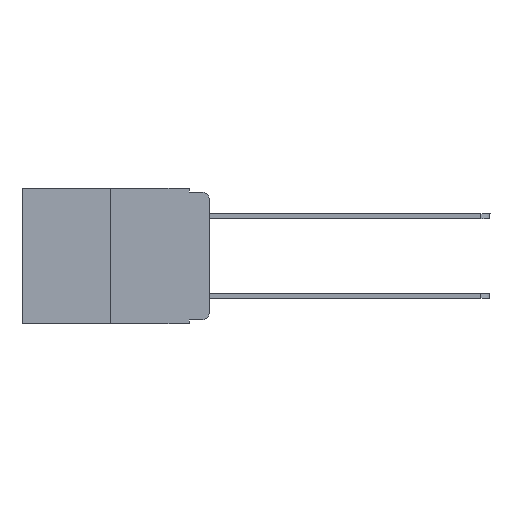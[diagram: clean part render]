
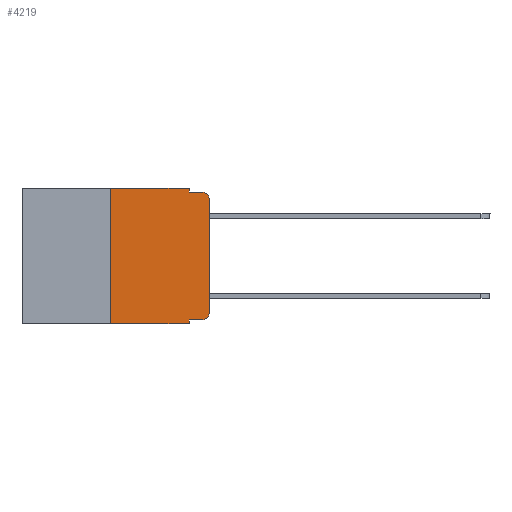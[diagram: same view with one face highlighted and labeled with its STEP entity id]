
A CAD part, left-side view. The second image highlights one B-rep face of the part: STEP entity #4219.
In plain terms, the highlighted planar face has unit normal (-1, 0, 0).
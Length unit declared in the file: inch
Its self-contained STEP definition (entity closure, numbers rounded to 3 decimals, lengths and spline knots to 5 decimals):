
#71 = LINE ( 'NONE', #4932, #4336 ) ;
#93 = ORIENTED_EDGE ( 'NONE', *, *, #1598, .T. ) ;
#201 = DIRECTION ( 'NONE',  ( 0., 0., -1. ) ) ;
#249 = LINE ( 'NONE', #7893, #498 ) ;
#393 = ORIENTED_EDGE ( 'NONE', *, *, #1706, .T. ) ;
#498 = VECTOR ( 'NONE', #201, 39.37008 ) ;
#511 = CARTESIAN_POINT ( 'NONE',  ( 0., 0., 0. ) ) ;
#796 = LINE ( 'NONE', #10152, #4245 ) ;
#922 = VECTOR ( 'NONE', #4833, 39.37008 ) ;
#968 = EDGE_CURVE ( 'NONE', #7519, #5631, #1173, .T. ) ;
#1173 = LINE ( 'NONE', #4576, #10884 ) ;
#1232 = VERTEX_POINT ( 'NONE', #2456 ) ;
#1481 = ORIENTED_EDGE ( 'NONE', *, *, #3990, .T. ) ;
#1534 = EDGE_CURVE ( 'NONE', #2841, #8915, #71, .T. ) ;
#1598 = EDGE_CURVE ( 'NONE', #9637, #6997, #3453, .T. ) ;
#1706 = EDGE_CURVE ( 'NONE', #8513, #3115, #5529, .T. ) ;
#1873 = DIRECTION ( 'NONE',  ( 0., 0., -1. ) ) ;
#2103 = VECTOR ( 'NONE', #5950, 39.37008 ) ;
#2187 = ORIENTED_EDGE ( 'NONE', *, *, #9310, .T. ) ;
#2409 = LINE ( 'NONE', #8347, #2103 ) ;
#2456 = CARTESIAN_POINT ( 'NONE',  ( 0., 0.051, -0.333 ) ) ;
#2657 = ORIENTED_EDGE ( 'NONE', *, *, #968, .F. ) ;
#2678 = AXIS2_PLACEMENT_3D ( 'NONE', #3198, #4904, #8282 ) ;
#2721 = AXIS2_PLACEMENT_3D ( 'NONE', #7747, #4549, #1873 ) ;
#2841 = VERTEX_POINT ( 'NONE', #9147 ) ;
#3019 = VECTOR ( 'NONE', #10771, 39.37008 ) ;
#3036 = LINE ( 'NONE', #511, #10265 ) ;
#3044 = LINE ( 'NONE', #4910, #3019 ) ;
#3115 = VERTEX_POINT ( 'NONE', #3872 ) ;
#3198 = CARTESIAN_POINT ( 'NONE',  ( 0., 0.473, 0. ) ) ;
#3229 = CARTESIAN_POINT ( 'NONE',  ( 0., 0.02, -0.03 ) ) ;
#3284 = DIRECTION ( 'NONE',  ( 0., 0., 1. ) ) ;
#3337 = CARTESIAN_POINT ( 'NONE',  ( 0., 0.051, -0.01 ) ) ;
#3453 = CIRCLE ( 'NONE', #9630, 0.02 ) ;
#3755 = ORIENTED_EDGE ( 'NONE', *, *, #6633, .T. ) ;
#3872 = CARTESIAN_POINT ( 'NONE',  ( 0., 0., -0.313 ) ) ;
#3990 = EDGE_CURVE ( 'NONE', #3115, #9637, #3036, .T. ) ;
#3995 = ORIENTED_EDGE ( 'NONE', *, *, #6628, .F. ) ;
#4008 = CARTESIAN_POINT ( 'NONE',  ( 0., 0.02, -0.01 ) ) ;
#4219 = ADVANCED_FACE ( 'NONE', ( #7389 ), #10763, .F. ) ;
#4245 = VECTOR ( 'NONE', #5728, 39.37008 ) ;
#4285 = CARTESIAN_POINT ( 'NONE',  ( 0., 0.25, 0. ) ) ;
#4336 = VECTOR ( 'NONE', #3284, 39.37008 ) ;
#4499 = ORIENTED_EDGE ( 'NONE', *, *, #1534, .F. ) ;
#4549 = DIRECTION ( 'NONE',  ( -1., 0., 0. ) ) ;
#4576 = CARTESIAN_POINT ( 'NONE',  ( 0., 0.051, 0. ) ) ;
#4583 = ORIENTED_EDGE ( 'NONE', *, *, #9629, .F. ) ;
#4687 = CARTESIAN_POINT ( 'NONE',  ( 0., 0.051, -0.343 ) ) ;
#4833 = DIRECTION ( 'NONE',  ( 0., -1., 0. ) ) ;
#4904 = DIRECTION ( 'NONE',  ( 1., 0., 0. ) ) ;
#4910 = CARTESIAN_POINT ( 'NONE',  ( 0., 0.473, -0.343 ) ) ;
#4932 = CARTESIAN_POINT ( 'NONE',  ( 0., 0.25, 0. ) ) ;
#4986 = ORIENTED_EDGE ( 'NONE', *, *, #5750, .F. ) ;
#5529 = CIRCLE ( 'NONE', #2721, 0.02 ) ;
#5631 = VERTEX_POINT ( 'NONE', #3337 ) ;
#5656 = CARTESIAN_POINT ( 'NONE',  ( 0., 0.473, 0. ) ) ;
#5728 = DIRECTION ( 'NONE',  ( 0., -1., 0. ) ) ;
#5750 = EDGE_CURVE ( 'NONE', #8915, #7519, #9853, .T. ) ;
#5950 = DIRECTION ( 'NONE',  ( 0., -1., 0. ) ) ;
#6335 = DIRECTION ( 'NONE',  ( 0., 0., 1. ) ) ;
#6598 = DIRECTION ( 'NONE',  ( 0., 0., -1. ) ) ;
#6628 = EDGE_CURVE ( 'NONE', #5631, #6997, #2409, .T. ) ;
#6633 = EDGE_CURVE ( 'NONE', #1232, #8513, #796, .T. ) ;
#6997 = VERTEX_POINT ( 'NONE', #4008 ) ;
#7389 = FACE_OUTER_BOUND ( 'NONE', #10640, .T. ) ;
#7519 = VERTEX_POINT ( 'NONE', #7578 ) ;
#7578 = CARTESIAN_POINT ( 'NONE',  ( 0., 0.051, 0. ) ) ;
#7747 = CARTESIAN_POINT ( 'NONE',  ( 0., 0.02, -0.313 ) ) ;
#7893 = CARTESIAN_POINT ( 'NONE',  ( 0., 0.051, 0. ) ) ;
#8282 = DIRECTION ( 'NONE',  ( 0., 0., -1. ) ) ;
#8347 = CARTESIAN_POINT ( 'NONE',  ( 0., 0.051, -0.01 ) ) ;
#8513 = VERTEX_POINT ( 'NONE', #9488 ) ;
#8616 = DIRECTION ( 'NONE',  ( 0., 0., -1. ) ) ;
#8739 = CARTESIAN_POINT ( 'NONE',  ( 0., 0., -0.03 ) ) ;
#8915 = VERTEX_POINT ( 'NONE', #4285 ) ;
#9147 = CARTESIAN_POINT ( 'NONE',  ( 0., 0.25, -0.343 ) ) ;
#9310 = EDGE_CURVE ( 'NONE', #2841, #9828, #3044, .T. ) ;
#9488 = CARTESIAN_POINT ( 'NONE',  ( 0., 0.02, -0.333 ) ) ;
#9629 = EDGE_CURVE ( 'NONE', #1232, #9828, #249, .T. ) ;
#9630 = AXIS2_PLACEMENT_3D ( 'NONE', #3229, #10006, #6598 ) ;
#9637 = VERTEX_POINT ( 'NONE', #8739 ) ;
#9828 = VERTEX_POINT ( 'NONE', #4687 ) ;
#9853 = LINE ( 'NONE', #5656, #922 ) ;
#10006 = DIRECTION ( 'NONE',  ( -1., 0., 0. ) ) ;
#10152 = CARTESIAN_POINT ( 'NONE',  ( 0., 0.051, -0.333 ) ) ;
#10265 = VECTOR ( 'NONE', #6335, 39.37008 ) ;
#10640 = EDGE_LOOP ( 'NONE', ( #1481, #93, #3995, #2657, #4986, #4499, #2187, #4583, #3755, #393 ) ) ;
#10763 = PLANE ( 'NONE',  #2678 ) ;
#10771 = DIRECTION ( 'NONE',  ( 0., -1., 0. ) ) ;
#10884 = VECTOR ( 'NONE', #8616, 39.37008 ) ;
